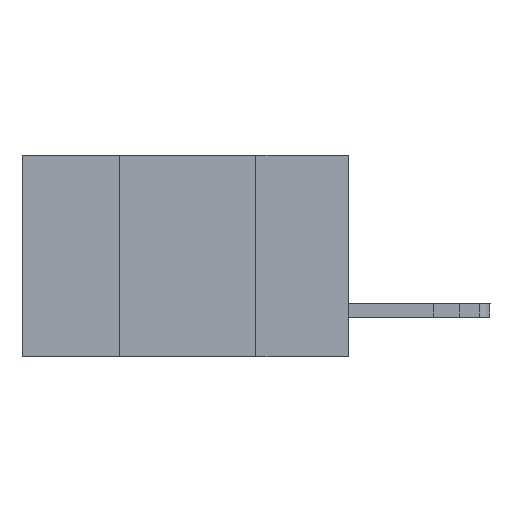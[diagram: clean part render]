
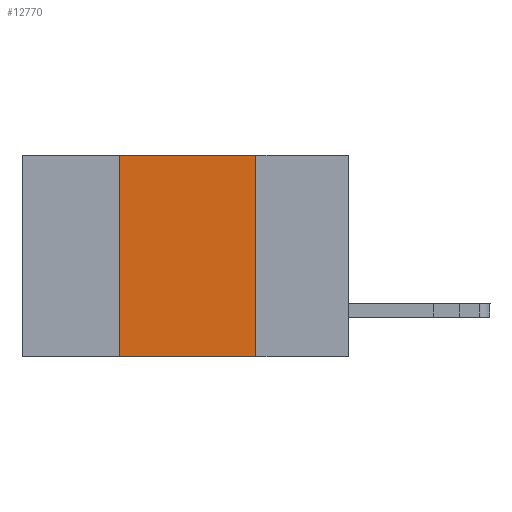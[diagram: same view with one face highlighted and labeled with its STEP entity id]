
A CAD part, left-side view. The second image highlights one B-rep face of the part: STEP entity #12770.
In plain terms, the highlighted planar face has unit normal (-1, 0, 0).
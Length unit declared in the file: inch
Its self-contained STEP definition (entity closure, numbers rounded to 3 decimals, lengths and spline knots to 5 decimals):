
#760 = CARTESIAN_POINT ( 'NONE',  ( 0., 0.17, 0. ) ) ;
#1370 = ORIENTED_EDGE ( 'NONE', *, *, #14657, .F. ) ;
#1406 = CARTESIAN_POINT ( 'NONE',  ( 0., 0.6, 0. ) ) ;
#1742 = VECTOR ( 'NONE', #5502, 39.37008 ) ;
#1841 = CARTESIAN_POINT ( 'NONE',  ( 0., 0.17, -0.37 ) ) ;
#2458 = VECTOR ( 'NONE', #7279, 39.37008 ) ;
#2514 = CARTESIAN_POINT ( 'NONE',  ( 0., 0.17, -0.37 ) ) ;
#2643 = CARTESIAN_POINT ( 'NONE',  ( 0., 0.42, -0.37 ) ) ;
#2858 = DIRECTION ( 'NONE',  ( 0., 0., 1. ) ) ;
#2964 = DIRECTION ( 'NONE',  ( 0., 0., -1. ) ) ;
#3054 = CARTESIAN_POINT ( 'NONE',  ( 0., 0.42, 0. ) ) ;
#3268 = CARTESIAN_POINT ( 'NONE',  ( 0., 0.42, -0.37 ) ) ;
#3947 = DIRECTION ( 'NONE',  ( 0., 0., -1. ) ) ;
#5502 = DIRECTION ( 'NONE',  ( 0., -1., 0. ) ) ;
#6011 = VECTOR ( 'NONE', #2858, 39.37008 ) ;
#6119 = EDGE_CURVE ( 'NONE', #12964, #15500, #19603, .T. ) ;
#7061 = CARTESIAN_POINT ( 'NONE',  ( 0., 0.6, -0.37 ) ) ;
#7272 = LINE ( 'NONE', #2514, #14125 ) ;
#7279 = DIRECTION ( 'NONE',  ( 0., -1., 0. ) ) ;
#9029 = LINE ( 'NONE', #10166, #2458 ) ;
#9367 = DIRECTION ( 'NONE',  ( 1., 0., 0. ) ) ;
#9956 = EDGE_CURVE ( 'NONE', #13330, #15500, #7272, .T. ) ;
#9985 = EDGE_LOOP ( 'NONE', ( #12522, #1370, #17977, #13967 ) ) ;
#10166 = CARTESIAN_POINT ( 'NONE',  ( 0., 0.6, 0. ) ) ;
#12522 = ORIENTED_EDGE ( 'NONE', *, *, #9956, .F. ) ;
#12734 = EDGE_CURVE ( 'NONE', #12964, #18851, #13950, .T. ) ;
#12770 = ADVANCED_FACE ( 'NONE', ( #17144 ), #17249, .F. ) ;
#12964 = VERTEX_POINT ( 'NONE', #2643 ) ;
#13330 = VERTEX_POINT ( 'NONE', #760 ) ;
#13950 = LINE ( 'NONE', #3268, #6011 ) ;
#13967 = ORIENTED_EDGE ( 'NONE', *, *, #6119, .T. ) ;
#14125 = VECTOR ( 'NONE', #3947, 39.37008 ) ;
#14657 = EDGE_CURVE ( 'NONE', #18851, #13330, #9029, .T. ) ;
#15500 = VERTEX_POINT ( 'NONE', #1841 ) ;
#17144 = FACE_OUTER_BOUND ( 'NONE', #9985, .T. ) ;
#17249 = PLANE ( 'NONE',  #20237 ) ;
#17977 = ORIENTED_EDGE ( 'NONE', *, *, #12734, .F. ) ;
#18851 = VERTEX_POINT ( 'NONE', #3054 ) ;
#19603 = LINE ( 'NONE', #7061, #1742 ) ;
#20237 = AXIS2_PLACEMENT_3D ( 'NONE', #1406, #9367, #2964 ) ;
